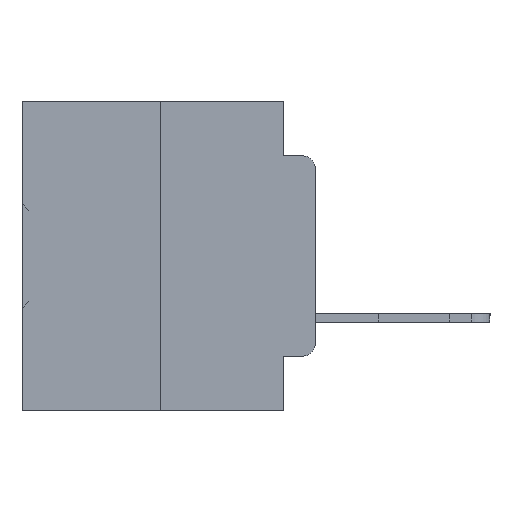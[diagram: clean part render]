
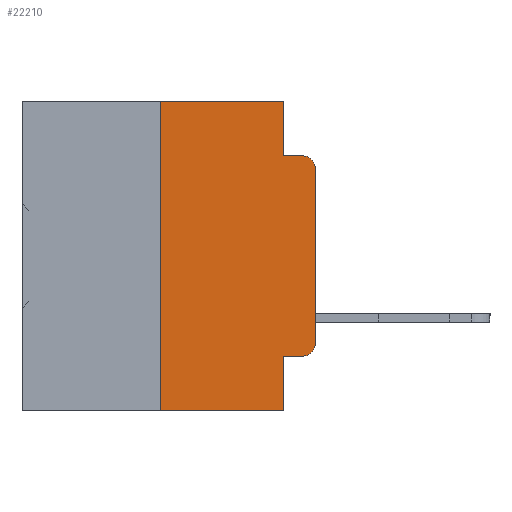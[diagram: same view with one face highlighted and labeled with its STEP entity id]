
A CAD part, left-side view. The second image highlights one B-rep face of the part: STEP entity #22210.
In plain terms, the highlighted planar face has unit normal (-1, 0, 0).
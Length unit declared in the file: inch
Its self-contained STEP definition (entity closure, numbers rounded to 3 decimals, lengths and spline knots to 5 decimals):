
#20 = CARTESIAN_POINT ( 'NONE',  ( 0., 0.051, -0.5 ) ) ;
#395 = EDGE_CURVE ( 'NONE', #1652, #4845, #34063, .T. ) ;
#489 = DIRECTION ( 'NONE',  ( 0., -1., 0. ) ) ;
#1325 = PLANE ( 'NONE',  #30493 ) ;
#1652 = VERTEX_POINT ( 'NONE', #4694 ) ;
#1730 = CARTESIAN_POINT ( 'NONE',  ( 0., 0.051, 0. ) ) ;
#1798 = DIRECTION ( 'NONE',  ( 0., -1., 0. ) ) ;
#1970 = DIRECTION ( 'NONE',  ( 0., -1., 0. ) ) ;
#2239 = DIRECTION ( 'NONE',  ( -1., 0., 0. ) ) ;
#3135 = EDGE_CURVE ( 'NONE', #25205, #29977, #28320, .T. ) ;
#3206 = CARTESIAN_POINT ( 'NONE',  ( 0., 0.25, 0. ) ) ;
#3222 = VERTEX_POINT ( 'NONE', #13473 ) ;
#3865 = EDGE_CURVE ( 'NONE', #15958, #3222, #23190, .T. ) ;
#4133 = DIRECTION ( 'NONE',  ( 0., 0., 1. ) ) ;
#4478 = CARTESIAN_POINT ( 'NONE',  ( 0., 0.051, 0. ) ) ;
#4694 = CARTESIAN_POINT ( 'NONE',  ( 0., 0.051, -0.4115 ) ) ;
#4845 = VERTEX_POINT ( 'NONE', #6340 ) ;
#5110 = VERTEX_POINT ( 'NONE', #22361 ) ;
#5929 = VECTOR ( 'NONE', #489, 39.37008 ) ;
#6340 = CARTESIAN_POINT ( 'NONE',  ( 0., 0.02, -0.4115 ) ) ;
#6360 = EDGE_CURVE ( 'NONE', #4845, #22949, #37776, .T. ) ;
#6582 = EDGE_LOOP ( 'NONE', ( #28471, #19199, #23443, #34555, #26321, #16518, #11516, #12939, #13403, #30624 ) ) ;
#6587 = EDGE_CURVE ( 'NONE', #12076, #5110, #18297, .T. ) ;
#7285 = DIRECTION ( 'NONE',  ( 1., 0., 0. ) ) ;
#8009 = VECTOR ( 'NONE', #1970, 39.37008 ) ;
#8020 = LINE ( 'NONE', #14614, #22048 ) ;
#11053 = DIRECTION ( 'NONE',  ( 0., -1., 0. ) ) ;
#11516 = ORIENTED_EDGE ( 'NONE', *, *, #17764, .T. ) ;
#12076 = VERTEX_POINT ( 'NONE', #16274 ) ;
#12939 = ORIENTED_EDGE ( 'NONE', *, *, #17027, .F. ) ;
#13403 = ORIENTED_EDGE ( 'NONE', *, *, #395, .T. ) ;
#13473 = CARTESIAN_POINT ( 'NONE',  ( 0., 0.051, -0.0885 ) ) ;
#13808 = LINE ( 'NONE', #24196, #5929 ) ;
#14614 = CARTESIAN_POINT ( 'NONE',  ( 0., 0., 0. ) ) ;
#14980 = LINE ( 'NONE', #37203, #8009 ) ;
#15877 = DIRECTION ( 'NONE',  ( -1., 0., 0. ) ) ;
#15958 = VERTEX_POINT ( 'NONE', #36739 ) ;
#16274 = CARTESIAN_POINT ( 'NONE',  ( 0., 0., -0.1085 ) ) ;
#16518 = ORIENTED_EDGE ( 'NONE', *, *, #3135, .F. ) ;
#17027 = EDGE_CURVE ( 'NONE', #1652, #17967, #34987, .T. ) ;
#17764 = EDGE_CURVE ( 'NONE', #25205, #17967, #14980, .T. ) ;
#17967 = VERTEX_POINT ( 'NONE', #20 ) ;
#18297 = CIRCLE ( 'NONE', #20746, 0.02 ) ;
#18491 = FACE_OUTER_BOUND ( 'NONE', #6582, .T. ) ;
#19199 = ORIENTED_EDGE ( 'NONE', *, *, #6587, .T. ) ;
#19234 = VECTOR ( 'NONE', #37128, 39.37008 ) ;
#20050 = CARTESIAN_POINT ( 'NONE',  ( 0., 0.02, -0.1085 ) ) ;
#20557 = EDGE_CURVE ( 'NONE', #3222, #5110, #38009, .T. ) ;
#20641 = DIRECTION ( 'NONE',  ( 0., 0., 1. ) ) ;
#20746 = AXIS2_PLACEMENT_3D ( 'NONE', #20050, #2239, #23070 ) ;
#21638 = CARTESIAN_POINT ( 'NONE',  ( 0., 0., -0.3915 ) ) ;
#22048 = VECTOR ( 'NONE', #20641, 39.37008 ) ;
#22167 = CARTESIAN_POINT ( 'NONE',  ( 0., 0.473, 0. ) ) ;
#22210 = ADVANCED_FACE ( 'NONE', ( #18491 ), #1325, .F. ) ;
#22361 = CARTESIAN_POINT ( 'NONE',  ( 0., 0.02, -0.0885 ) ) ;
#22710 = DIRECTION ( 'NONE',  ( 0., 0., -1. ) ) ;
#22949 = VERTEX_POINT ( 'NONE', #21638 ) ;
#23070 = DIRECTION ( 'NONE',  ( 0., 0., -1. ) ) ;
#23190 = LINE ( 'NONE', #1730, #37910 ) ;
#23443 = ORIENTED_EDGE ( 'NONE', *, *, #20557, .F. ) ;
#23496 = AXIS2_PLACEMENT_3D ( 'NONE', #33647, #15877, #36593 ) ;
#24196 = CARTESIAN_POINT ( 'NONE',  ( 0., 0.473, 0. ) ) ;
#24958 = CARTESIAN_POINT ( 'NONE',  ( 0., 0.25, 0. ) ) ;
#25205 = VERTEX_POINT ( 'NONE', #35901 ) ;
#25334 = VECTOR ( 'NONE', #1798, 39.37008 ) ;
#25479 = CARTESIAN_POINT ( 'NONE',  ( 0., 0.051, -0.4115 ) ) ;
#26321 = ORIENTED_EDGE ( 'NONE', *, *, #34133, .F. ) ;
#27282 = EDGE_CURVE ( 'NONE', #22949, #12076, #8020, .T. ) ;
#28095 = DIRECTION ( 'NONE',  ( 0., 0., -1. ) ) ;
#28320 = LINE ( 'NONE', #24958, #35221 ) ;
#28471 = ORIENTED_EDGE ( 'NONE', *, *, #27282, .T. ) ;
#28846 = CARTESIAN_POINT ( 'NONE',  ( 0., 0.051, -0.0885 ) ) ;
#29977 = VERTEX_POINT ( 'NONE', #3206 ) ;
#30209 = VECTOR ( 'NONE', #11053, 39.37008 ) ;
#30493 = AXIS2_PLACEMENT_3D ( 'NONE', #22167, #7285, #28095 ) ;
#30624 = ORIENTED_EDGE ( 'NONE', *, *, #6360, .T. ) ;
#33647 = CARTESIAN_POINT ( 'NONE',  ( 0., 0.02, -0.3915 ) ) ;
#34063 = LINE ( 'NONE', #25479, #25334 ) ;
#34133 = EDGE_CURVE ( 'NONE', #29977, #15958, #13808, .T. ) ;
#34555 = ORIENTED_EDGE ( 'NONE', *, *, #3865, .F. ) ;
#34987 = LINE ( 'NONE', #4478, #19234 ) ;
#35221 = VECTOR ( 'NONE', #4133, 39.37008 ) ;
#35901 = CARTESIAN_POINT ( 'NONE',  ( 0., 0.25, -0.5 ) ) ;
#36593 = DIRECTION ( 'NONE',  ( 0., 0., -1. ) ) ;
#36739 = CARTESIAN_POINT ( 'NONE',  ( 0., 0.051, 0. ) ) ;
#37128 = DIRECTION ( 'NONE',  ( 0., 0., -1. ) ) ;
#37203 = CARTESIAN_POINT ( 'NONE',  ( 0., 0.473, -0.5 ) ) ;
#37776 = CIRCLE ( 'NONE', #23496, 0.02 ) ;
#37910 = VECTOR ( 'NONE', #22710, 39.37008 ) ;
#38009 = LINE ( 'NONE', #28846, #30209 ) ;
